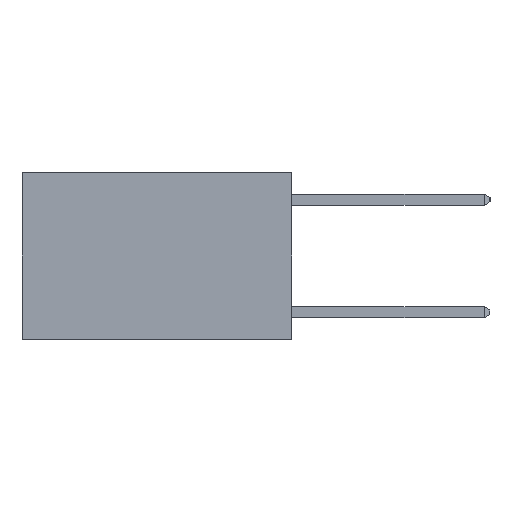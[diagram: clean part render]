
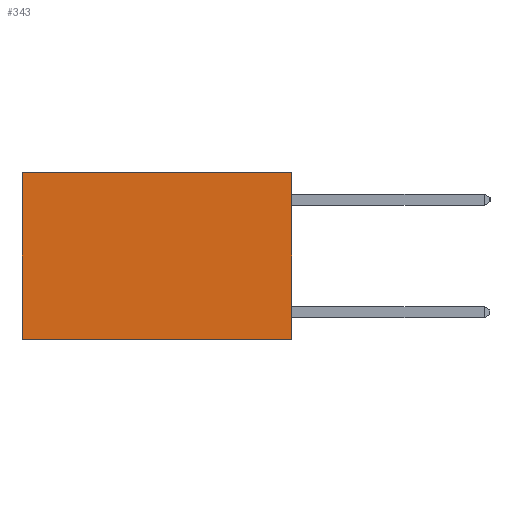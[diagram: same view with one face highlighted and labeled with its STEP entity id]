
A CAD part, left-side view. The second image highlights one B-rep face of the part: STEP entity #343.
In plain terms, the highlighted planar face has unit normal (-1, 0, 0).
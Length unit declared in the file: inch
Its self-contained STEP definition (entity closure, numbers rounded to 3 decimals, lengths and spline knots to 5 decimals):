
#170 = EDGE_CURVE ( 'NONE', #4728, #440, #2732, .T. ) ;
#298 = VECTOR ( 'NONE', #9854, 39.37008 ) ;
#343 = ADVANCED_FACE ( 'NONE', ( #10516 ), #6973, .F. ) ;
#440 = VERTEX_POINT ( 'NONE', #5400 ) ;
#1997 = VECTOR ( 'NONE', #5682, 39.37008 ) ;
#2732 = LINE ( 'NONE', #9896, #6880 ) ;
#3513 = ORIENTED_EDGE ( 'NONE', *, *, #5597, .F. ) ;
#3721 = LINE ( 'NONE', #5670, #6189 ) ;
#3774 = EDGE_CURVE ( 'NONE', #440, #8839, #3721, .T. ) ;
#4428 = ORIENTED_EDGE ( 'NONE', *, *, #5422, .F. ) ;
#4479 = CARTESIAN_POINT ( 'NONE',  ( 0.2625, 0.6, -0.37 ) ) ;
#4728 = VERTEX_POINT ( 'NONE', #5691 ) ;
#5400 = CARTESIAN_POINT ( 'NONE',  ( 0.2625, 0.6, 0. ) ) ;
#5422 = EDGE_CURVE ( 'NONE', #7339, #8839, #8581, .T. ) ;
#5597 = EDGE_CURVE ( 'NONE', #4728, #7339, #7059, .T. ) ;
#5633 = DIRECTION ( 'NONE',  ( 0., 0., -1. ) ) ;
#5670 = CARTESIAN_POINT ( 'NONE',  ( 0.2625, 0.6, 0. ) ) ;
#5682 = DIRECTION ( 'NONE',  ( 0., 1., 0. ) ) ;
#5691 = CARTESIAN_POINT ( 'NONE',  ( 0.2625, 0., 0. ) ) ;
#5758 = ORIENTED_EDGE ( 'NONE', *, *, #170, .T. ) ;
#5793 = EDGE_LOOP ( 'NONE', ( #10751, #4428, #3513, #5758 ) ) ;
#5904 = CARTESIAN_POINT ( 'NONE',  ( 0.2625, 0., -0.37 ) ) ;
#6189 = VECTOR ( 'NONE', #5633, 39.37008 ) ;
#6880 = VECTOR ( 'NONE', #9830, 39.37008 ) ;
#6930 = DIRECTION ( 'NONE',  ( 0., 0., -1. ) ) ;
#6947 = DIRECTION ( 'NONE',  ( 1., 0., 0. ) ) ;
#6973 = PLANE ( 'NONE',  #10001 ) ;
#6988 = CARTESIAN_POINT ( 'NONE',  ( 0.2625, 0., 0. ) ) ;
#7059 = LINE ( 'NONE', #9055, #298 ) ;
#7339 = VERTEX_POINT ( 'NONE', #5904 ) ;
#8581 = LINE ( 'NONE', #8884, #1997 ) ;
#8839 = VERTEX_POINT ( 'NONE', #4479 ) ;
#8884 = CARTESIAN_POINT ( 'NONE',  ( 0.2625, 0., -0.37 ) ) ;
#9055 = CARTESIAN_POINT ( 'NONE',  ( 0.2625, 0., 0. ) ) ;
#9830 = DIRECTION ( 'NONE',  ( 0., 1., 0. ) ) ;
#9854 = DIRECTION ( 'NONE',  ( 0., 0., -1. ) ) ;
#9896 = CARTESIAN_POINT ( 'NONE',  ( 0.2625, 0., 0. ) ) ;
#10001 = AXIS2_PLACEMENT_3D ( 'NONE', #6988, #6947, #6930 ) ;
#10516 = FACE_OUTER_BOUND ( 'NONE', #5793, .T. ) ;
#10751 = ORIENTED_EDGE ( 'NONE', *, *, #3774, .T. ) ;
